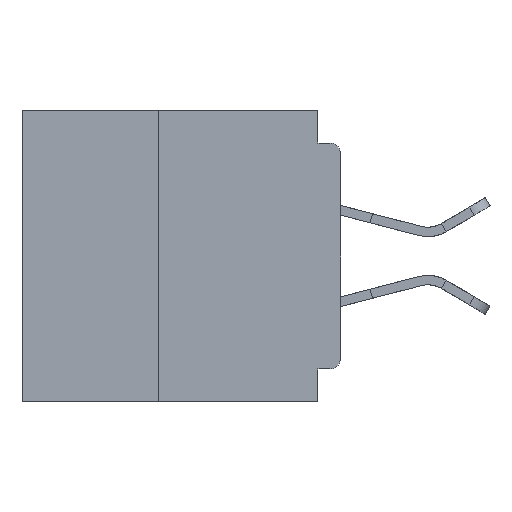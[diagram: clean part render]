
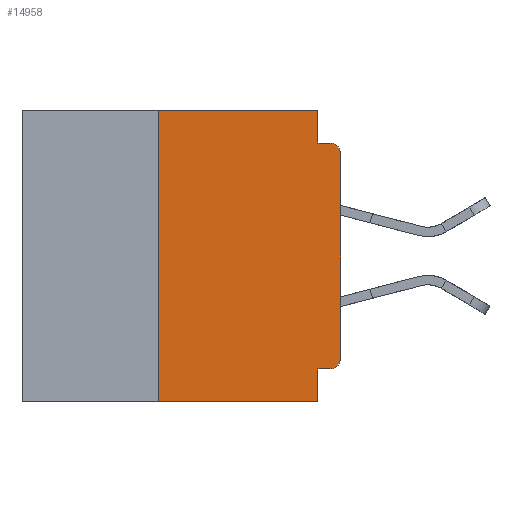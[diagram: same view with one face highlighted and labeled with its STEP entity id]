
A CAD part, left-side view. The second image highlights one B-rep face of the part: STEP entity #14958.
In plain terms, the highlighted planar face has unit normal (-1, 0, 0).
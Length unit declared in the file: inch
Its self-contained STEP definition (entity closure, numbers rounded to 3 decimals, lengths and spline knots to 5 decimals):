
#1379 = EDGE_CURVE ( 'NONE', #15145, #45864, #12951, .T. ) ;
#1587 = CARTESIAN_POINT ( 'NONE',  ( 0., 0., -0.355 ) ) ;
#1872 = DIRECTION ( 'NONE',  ( 0., 0., -1. ) ) ;
#2806 = CARTESIAN_POINT ( 'NONE',  ( 0., 0., -0.34 ) ) ;
#3568 = CARTESIAN_POINT ( 'NONE',  ( 0., 0., -0.045 ) ) ;
#4343 = ORIENTED_EDGE ( 'NONE', *, *, #33660, .F. ) ;
#4391 = DIRECTION ( 'NONE',  ( 0., 0., 1. ) ) ;
#4740 = PLANE ( 'NONE',  #43190 ) ;
#4800 = CARTESIAN_POINT ( 'NONE',  ( 0., 0.015, -0.06 ) ) ;
#4916 = LINE ( 'NONE', #39223, #45017 ) ;
#5037 = VERTEX_POINT ( 'NONE', #30738 ) ;
#5739 = CARTESIAN_POINT ( 'NONE',  ( 0., 0.015, -0.355 ) ) ;
#6223 = VERTEX_POINT ( 'NONE', #18768 ) ;
#6911 = CARTESIAN_POINT ( 'NONE',  ( 0., 0.25, -0.4 ) ) ;
#7252 = LINE ( 'NONE', #46946, #27969 ) ;
#7881 = VERTEX_POINT ( 'NONE', #6911 ) ;
#8262 = CARTESIAN_POINT ( 'NONE',  ( 0., 0., -0.06 ) ) ;
#8684 = DIRECTION ( 'NONE',  ( 0., 0., -1. ) ) ;
#8685 = EDGE_CURVE ( 'NONE', #7881, #24263, #7252, .T. ) ;
#10511 = ORIENTED_EDGE ( 'NONE', *, *, #41384, .F. ) ;
#10955 = LINE ( 'NONE', #3568, #40785 ) ;
#11340 = LINE ( 'NONE', #1587, #39956 ) ;
#12283 = EDGE_CURVE ( 'NONE', #16584, #6223, #32675, .T. ) ;
#12559 = DIRECTION ( 'NONE',  ( 0., 0., -1. ) ) ;
#12951 = CIRCLE ( 'NONE', #28108, 0.015 ) ;
#13500 = CARTESIAN_POINT ( 'NONE',  ( 0., 0., 0. ) ) ;
#13546 = LINE ( 'NONE', #22025, #30537 ) ;
#14550 = VERTEX_POINT ( 'NONE', #44862 ) ;
#14958 = ADVANCED_FACE ( 'NONE', ( #48809 ), #4740, .F. ) ;
#15145 = VERTEX_POINT ( 'NONE', #5739 ) ;
#15256 = EDGE_CURVE ( 'NONE', #35006, #14550, #13546, .T. ) ;
#16092 = EDGE_CURVE ( 'NONE', #48485, #6223, #10955, .T. ) ;
#16584 = VERTEX_POINT ( 'NONE', #8262 ) ;
#16849 = EDGE_LOOP ( 'NONE', ( #35356, #26811, #40811, #10511, #28810, #33653, #32458, #19391, #4343, #23199 ) ) ;
#18768 = CARTESIAN_POINT ( 'NONE',  ( 0., 0.015, -0.045 ) ) ;
#19391 = ORIENTED_EDGE ( 'NONE', *, *, #42311, .F. ) ;
#20013 = LINE ( 'NONE', #23594, #39454 ) ;
#21146 = CARTESIAN_POINT ( 'NONE',  ( 0., 0.031, 0. ) ) ;
#22025 = CARTESIAN_POINT ( 'NONE',  ( 0., 0.437, 0. ) ) ;
#22401 = LINE ( 'NONE', #13500, #31508 ) ;
#22510 = VECTOR ( 'NONE', #1872, 39.37008 ) ;
#23199 = ORIENTED_EDGE ( 'NONE', *, *, #1379, .T. ) ;
#23594 = CARTESIAN_POINT ( 'NONE',  ( 0., 0.031, -0.4 ) ) ;
#23697 = DIRECTION ( 'NONE',  ( 0., -1., 0. ) ) ;
#24263 = VERTEX_POINT ( 'NONE', #46115 ) ;
#26811 = ORIENTED_EDGE ( 'NONE', *, *, #12283, .T. ) ;
#26886 = DIRECTION ( 'NONE',  ( 0., -1., 0. ) ) ;
#27969 = VECTOR ( 'NONE', #23697, 39.37008 ) ;
#28108 = AXIS2_PLACEMENT_3D ( 'NONE', #38374, #38260, #38309 ) ;
#28810 = ORIENTED_EDGE ( 'NONE', *, *, #15256, .F. ) ;
#30537 = VECTOR ( 'NONE', #41407, 39.37008 ) ;
#30721 = EDGE_CURVE ( 'NONE', #7881, #35006, #4916, .T. ) ;
#30738 = CARTESIAN_POINT ( 'NONE',  ( 0., 0.031, -0.355 ) ) ;
#31508 = VECTOR ( 'NONE', #36765, 39.37008 ) ;
#31907 = CARTESIAN_POINT ( 'NONE',  ( 0., 0.437, 0. ) ) ;
#31908 = EDGE_CURVE ( 'NONE', #45864, #16584, #22401, .T. ) ;
#31959 = DIRECTION ( 'NONE',  ( -1., 0., 0. ) ) ;
#32458 = ORIENTED_EDGE ( 'NONE', *, *, #8685, .T. ) ;
#32675 = CIRCLE ( 'NONE', #45061, 0.015 ) ;
#32693 = DIRECTION ( 'NONE',  ( 0., 1., 0. ) ) ;
#32850 = LINE ( 'NONE', #21146, #22510 ) ;
#33653 = ORIENTED_EDGE ( 'NONE', *, *, #30721, .F. ) ;
#33660 = EDGE_CURVE ( 'NONE', #15145, #5037, #11340, .T. ) ;
#34876 = CARTESIAN_POINT ( 'NONE',  ( 0., 0.031, -0.045 ) ) ;
#35006 = VERTEX_POINT ( 'NONE', #36166 ) ;
#35291 = DIRECTION ( 'NONE',  ( 0., 0., -1. ) ) ;
#35356 = ORIENTED_EDGE ( 'NONE', *, *, #31908, .T. ) ;
#35817 = DIRECTION ( 'NONE',  ( 1., 0., 0. ) ) ;
#36166 = CARTESIAN_POINT ( 'NONE',  ( 0., 0.25, 0. ) ) ;
#36765 = DIRECTION ( 'NONE',  ( 0., 0., 1. ) ) ;
#38260 = DIRECTION ( 'NONE',  ( -1., 0., 0. ) ) ;
#38309 = DIRECTION ( 'NONE',  ( 0., 0., -1. ) ) ;
#38374 = CARTESIAN_POINT ( 'NONE',  ( 0., 0.015, -0.34 ) ) ;
#39223 = CARTESIAN_POINT ( 'NONE',  ( 0., 0.25, -0.4 ) ) ;
#39454 = VECTOR ( 'NONE', #35291, 39.37008 ) ;
#39956 = VECTOR ( 'NONE', #32693, 39.37008 ) ;
#40785 = VECTOR ( 'NONE', #26886, 39.37008 ) ;
#40811 = ORIENTED_EDGE ( 'NONE', *, *, #16092, .F. ) ;
#41384 = EDGE_CURVE ( 'NONE', #14550, #48485, #32850, .T. ) ;
#41407 = DIRECTION ( 'NONE',  ( 0., -1., 0. ) ) ;
#42311 = EDGE_CURVE ( 'NONE', #5037, #24263, #20013, .T. ) ;
#43190 = AXIS2_PLACEMENT_3D ( 'NONE', #31907, #35817, #12559 ) ;
#44862 = CARTESIAN_POINT ( 'NONE',  ( 0., 0.031, 0. ) ) ;
#45017 = VECTOR ( 'NONE', #4391, 39.37008 ) ;
#45061 = AXIS2_PLACEMENT_3D ( 'NONE', #4800, #31959, #8684 ) ;
#45864 = VERTEX_POINT ( 'NONE', #2806 ) ;
#46115 = CARTESIAN_POINT ( 'NONE',  ( 0., 0.031, -0.4 ) ) ;
#46946 = CARTESIAN_POINT ( 'NONE',  ( 0., 0.437, -0.4 ) ) ;
#48485 = VERTEX_POINT ( 'NONE', #34876 ) ;
#48809 = FACE_OUTER_BOUND ( 'NONE', #16849, .T. ) ;
